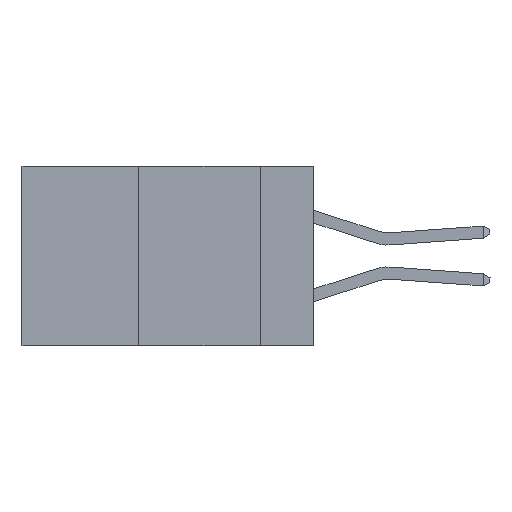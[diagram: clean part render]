
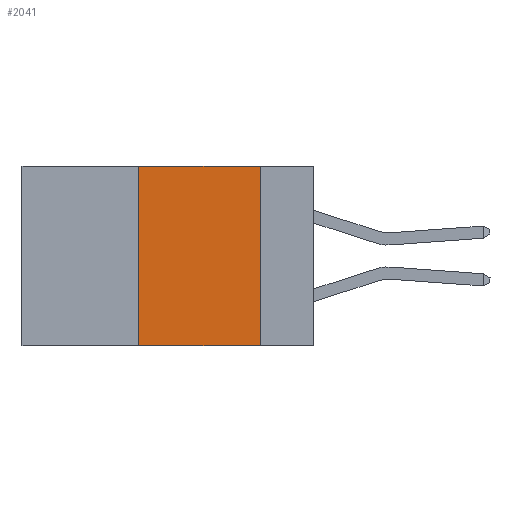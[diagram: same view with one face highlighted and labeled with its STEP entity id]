
A CAD part, left-side view. The second image highlights one B-rep face of the part: STEP entity #2041.
In plain terms, the highlighted planar face has unit normal (-1, 0, 0).
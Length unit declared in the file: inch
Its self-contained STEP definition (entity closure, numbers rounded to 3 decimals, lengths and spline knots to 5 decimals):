
#494 = DIRECTION ( 'NONE',  ( 1., 0., 0. ) ) ;
#2041 = ADVANCED_FACE ( 'NONE', ( #21177 ), #16166, .F. ) ;
#3543 = CARTESIAN_POINT ( 'NONE',  ( 0., 0.6, 0. ) ) ;
#4231 = VERTEX_POINT ( 'NONE', #25210 ) ;
#4589 = EDGE_CURVE ( 'NONE', #9844, #23735, #17542, .T. ) ;
#4678 = ORIENTED_EDGE ( 'NONE', *, *, #21793, .F. ) ;
#6128 = EDGE_CURVE ( 'NONE', #9844, #4231, #21282, .T. ) ;
#7255 = CARTESIAN_POINT ( 'NONE',  ( 0., 0.11, 0. ) ) ;
#7385 = CARTESIAN_POINT ( 'NONE',  ( 0., 0.6, -0.37 ) ) ;
#8399 = LINE ( 'NONE', #7255, #28520 ) ;
#8439 = DIRECTION ( 'NONE',  ( 0., -1., 0. ) ) ;
#9330 = CARTESIAN_POINT ( 'NONE',  ( 0., 0.11, 0. ) ) ;
#9394 = VECTOR ( 'NONE', #17473, 39.37008 ) ;
#9844 = VERTEX_POINT ( 'NONE', #23265 ) ;
#9991 = CARTESIAN_POINT ( 'NONE',  ( 0., 0.36, 0. ) ) ;
#10394 = VECTOR ( 'NONE', #8439, 39.37008 ) ;
#11225 = EDGE_CURVE ( 'NONE', #23735, #21563, #26986, .T. ) ;
#12947 = CARTESIAN_POINT ( 'NONE',  ( 0., 0.36, 0. ) ) ;
#14322 = DIRECTION ( 'NONE',  ( 0., -1., 0. ) ) ;
#16166 = PLANE ( 'NONE',  #22794 ) ;
#17473 = DIRECTION ( 'NONE',  ( 0., 0., 1. ) ) ;
#17542 = LINE ( 'NONE', #12947, #9394 ) ;
#18618 = DIRECTION ( 'NONE',  ( 0., 0., -1. ) ) ;
#18721 = CARTESIAN_POINT ( 'NONE',  ( 0., 0.6, 0. ) ) ;
#20664 = EDGE_LOOP ( 'NONE', ( #4678, #26647, #23798, #28463 ) ) ;
#21177 = FACE_OUTER_BOUND ( 'NONE', #20664, .T. ) ;
#21282 = LINE ( 'NONE', #7385, #29019 ) ;
#21563 = VERTEX_POINT ( 'NONE', #9330 ) ;
#21793 = EDGE_CURVE ( 'NONE', #21563, #4231, #8399, .T. ) ;
#22794 = AXIS2_PLACEMENT_3D ( 'NONE', #18721, #494, #18618 ) ;
#23265 = CARTESIAN_POINT ( 'NONE',  ( 0., 0.36, -0.37 ) ) ;
#23735 = VERTEX_POINT ( 'NONE', #9991 ) ;
#23798 = ORIENTED_EDGE ( 'NONE', *, *, #4589, .F. ) ;
#23852 = DIRECTION ( 'NONE',  ( 0., 0., -1. ) ) ;
#25210 = CARTESIAN_POINT ( 'NONE',  ( 0., 0.11, -0.37 ) ) ;
#26647 = ORIENTED_EDGE ( 'NONE', *, *, #11225, .F. ) ;
#26986 = LINE ( 'NONE', #3543, #10394 ) ;
#28463 = ORIENTED_EDGE ( 'NONE', *, *, #6128, .T. ) ;
#28520 = VECTOR ( 'NONE', #23852, 39.37008 ) ;
#29019 = VECTOR ( 'NONE', #14322, 39.37008 ) ;
